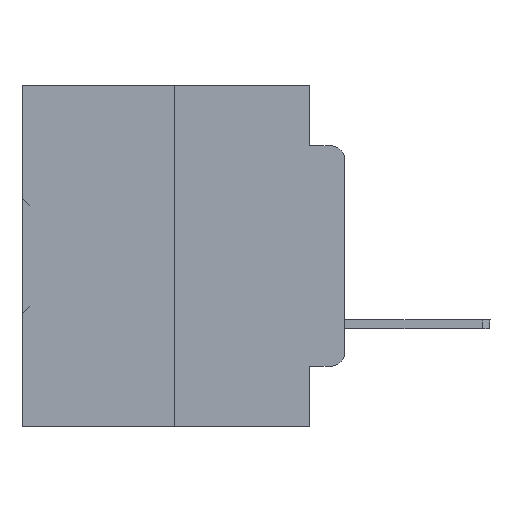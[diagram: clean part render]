
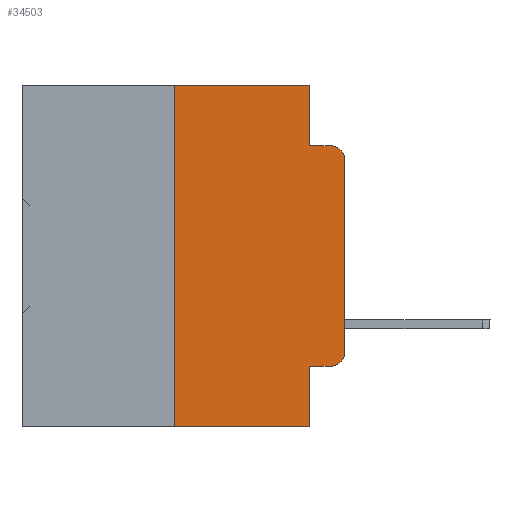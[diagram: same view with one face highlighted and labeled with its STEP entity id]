
A CAD part, left-side view. The second image highlights one B-rep face of the part: STEP entity #34503.
In plain terms, the highlighted planar face has unit normal (-1, 0, 0).
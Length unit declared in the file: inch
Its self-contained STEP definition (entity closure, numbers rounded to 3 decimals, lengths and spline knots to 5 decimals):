
#701 = ORIENTED_EDGE ( 'NONE', *, *, #27436, .F. ) ;
#724 = CARTESIAN_POINT ( 'NONE',  ( 0., 0.02, -0.3915 ) ) ;
#1161 = DIRECTION ( 'NONE',  ( 0., 0., -1. ) ) ;
#1396 = LINE ( 'NONE', #21501, #31558 ) ;
#1483 = VECTOR ( 'NONE', #16191, 39.37008 ) ;
#1488 = DIRECTION ( 'NONE',  ( 0., -1., 0. ) ) ;
#2055 = VECTOR ( 'NONE', #1161, 39.37008 ) ;
#2281 = DIRECTION ( 'NONE',  ( 0., 0., -1. ) ) ;
#2339 = VERTEX_POINT ( 'NONE', #37286 ) ;
#2682 = VERTEX_POINT ( 'NONE', #21313 ) ;
#2983 = CARTESIAN_POINT ( 'NONE',  ( 0., 0.02, -0.0885 ) ) ;
#3917 = FACE_OUTER_BOUND ( 'NONE', #8568, .T. ) ;
#4652 = ORIENTED_EDGE ( 'NONE', *, *, #20198, .F. ) ;
#5504 = PLANE ( 'NONE',  #36536 ) ;
#5909 = EDGE_CURVE ( 'NONE', #2339, #2682, #35851, .T. ) ;
#6045 = VERTEX_POINT ( 'NONE', #10705 ) ;
#6116 = CARTESIAN_POINT ( 'NONE',  ( 0., 0., 0. ) ) ;
#6690 = LINE ( 'NONE', #21895, #2055 ) ;
#7200 = CARTESIAN_POINT ( 'NONE',  ( 0., 0.051, -0.0885 ) ) ;
#7824 = VECTOR ( 'NONE', #12942, 39.37008 ) ;
#8142 = CARTESIAN_POINT ( 'NONE',  ( 0., 0., -0.1085 ) ) ;
#8568 = EDGE_LOOP ( 'NONE', ( #18275, #17423, #4652, #35795, #16291, #701, #12215, #36421, #14650, #18044 ) ) ;
#8889 = CARTESIAN_POINT ( 'NONE',  ( 0., 0.051, 0. ) ) ;
#9073 = DIRECTION ( 'NONE',  ( 0., 0., 1. ) ) ;
#9315 = LINE ( 'NONE', #7200, #25736 ) ;
#10705 = CARTESIAN_POINT ( 'NONE',  ( 0., 0.25, 0. ) ) ;
#10947 = AXIS2_PLACEMENT_3D ( 'NONE', #724, #23725, #18003 ) ;
#10956 = CARTESIAN_POINT ( 'NONE',  ( 0., 0., -0.3915 ) ) ;
#12031 = EDGE_CURVE ( 'NONE', #36303, #19259, #21187, .T. ) ;
#12055 = EDGE_CURVE ( 'NONE', #2682, #36303, #22095, .T. ) ;
#12215 = ORIENTED_EDGE ( 'NONE', *, *, #36188, .T. ) ;
#12942 = DIRECTION ( 'NONE',  ( 0., 0., -1. ) ) ;
#13432 = VERTEX_POINT ( 'NONE', #8889 ) ;
#13503 = DIRECTION ( 'NONE',  ( 0., -1., 0. ) ) ;
#14650 = ORIENTED_EDGE ( 'NONE', *, *, #5909, .T. ) ;
#14696 = LINE ( 'NONE', #18797, #28390 ) ;
#15415 = EDGE_CURVE ( 'NONE', #2339, #19431, #22880, .T. ) ;
#16070 = CARTESIAN_POINT ( 'NONE',  ( 0., 0.473, -0.5 ) ) ;
#16191 = DIRECTION ( 'NONE',  ( 0., -1., 0. ) ) ;
#16196 = CARTESIAN_POINT ( 'NONE',  ( 0., 0.051, -0.4115 ) ) ;
#16291 = ORIENTED_EDGE ( 'NONE', *, *, #20719, .F. ) ;
#17081 = CARTESIAN_POINT ( 'NONE',  ( 0., 0.25, -0.5 ) ) ;
#17423 = ORIENTED_EDGE ( 'NONE', *, *, #27577, .T. ) ;
#18003 = DIRECTION ( 'NONE',  ( 0., 0., -1. ) ) ;
#18044 = ORIENTED_EDGE ( 'NONE', *, *, #12055, .T. ) ;
#18275 = ORIENTED_EDGE ( 'NONE', *, *, #12031, .T. ) ;
#18605 = CARTESIAN_POINT ( 'NONE',  ( 0., 0.051, 0. ) ) ;
#18797 = CARTESIAN_POINT ( 'NONE',  ( 0., 0.473, 0. ) ) ;
#19222 = VERTEX_POINT ( 'NONE', #17081 ) ;
#19259 = VERTEX_POINT ( 'NONE', #8142 ) ;
#19431 = VERTEX_POINT ( 'NONE', #35440 ) ;
#19828 = VECTOR ( 'NONE', #9073, 39.37008 ) ;
#20198 = EDGE_CURVE ( 'NONE', #33062, #22813, #9315, .T. ) ;
#20620 = CIRCLE ( 'NONE', #36596, 0.02 ) ;
#20719 = EDGE_CURVE ( 'NONE', #6045, #13432, #14696, .T. ) ;
#21187 = LINE ( 'NONE', #6116, #19828 ) ;
#21313 = CARTESIAN_POINT ( 'NONE',  ( 0., 0.02, -0.4115 ) ) ;
#21386 = DIRECTION ( 'NONE',  ( 0., 0., 1. ) ) ;
#21501 = CARTESIAN_POINT ( 'NONE',  ( 0., 0.25, 0. ) ) ;
#21895 = CARTESIAN_POINT ( 'NONE',  ( 0., 0.051, 0. ) ) ;
#22095 = CIRCLE ( 'NONE', #10947, 0.02 ) ;
#22813 = VERTEX_POINT ( 'NONE', #2983 ) ;
#22880 = LINE ( 'NONE', #18605, #7824 ) ;
#23725 = DIRECTION ( 'NONE',  ( -1., 0., 0. ) ) ;
#24545 = DIRECTION ( 'NONE',  ( 0., 0., -1. ) ) ;
#25047 = DIRECTION ( 'NONE',  ( -1., 0., 0. ) ) ;
#25199 = CARTESIAN_POINT ( 'NONE',  ( 0., 0.051, -0.0885 ) ) ;
#25736 = VECTOR ( 'NONE', #31304, 39.37008 ) ;
#25796 = DIRECTION ( 'NONE',  ( 1., 0., 0. ) ) ;
#26635 = LINE ( 'NONE', #16070, #1483 ) ;
#27436 = EDGE_CURVE ( 'NONE', #19222, #6045, #1396, .T. ) ;
#27577 = EDGE_CURVE ( 'NONE', #19259, #22813, #20620, .T. ) ;
#28390 = VECTOR ( 'NONE', #13503, 39.37008 ) ;
#31304 = DIRECTION ( 'NONE',  ( 0., -1., 0. ) ) ;
#31558 = VECTOR ( 'NONE', #21386, 39.37008 ) ;
#31733 = VECTOR ( 'NONE', #1488, 39.37008 ) ;
#33062 = VERTEX_POINT ( 'NONE', #25199 ) ;
#33213 = CARTESIAN_POINT ( 'NONE',  ( 0., 0.02, -0.1085 ) ) ;
#34315 = EDGE_CURVE ( 'NONE', #13432, #33062, #6690, .T. ) ;
#34480 = CARTESIAN_POINT ( 'NONE',  ( 0., 0.473, 0. ) ) ;
#34503 = ADVANCED_FACE ( 'NONE', ( #3917 ), #5504, .F. ) ;
#35440 = CARTESIAN_POINT ( 'NONE',  ( 0., 0.051, -0.5 ) ) ;
#35795 = ORIENTED_EDGE ( 'NONE', *, *, #34315, .F. ) ;
#35851 = LINE ( 'NONE', #16196, #31733 ) ;
#36188 = EDGE_CURVE ( 'NONE', #19222, #19431, #26635, .T. ) ;
#36303 = VERTEX_POINT ( 'NONE', #10956 ) ;
#36421 = ORIENTED_EDGE ( 'NONE', *, *, #15415, .F. ) ;
#36536 = AXIS2_PLACEMENT_3D ( 'NONE', #34480, #25796, #2281 ) ;
#36596 = AXIS2_PLACEMENT_3D ( 'NONE', #33213, #25047, #24545 ) ;
#37286 = CARTESIAN_POINT ( 'NONE',  ( 0., 0.051, -0.4115 ) ) ;
